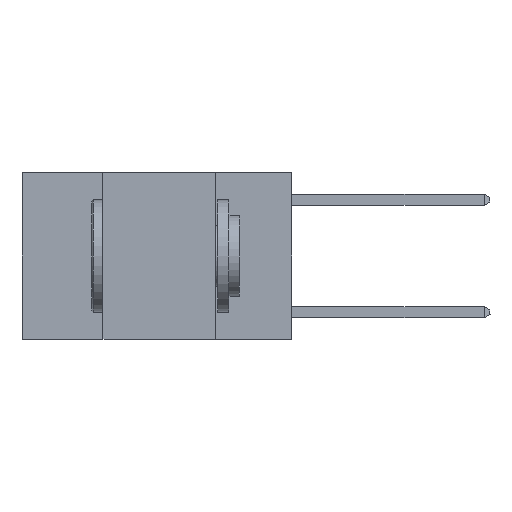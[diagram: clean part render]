
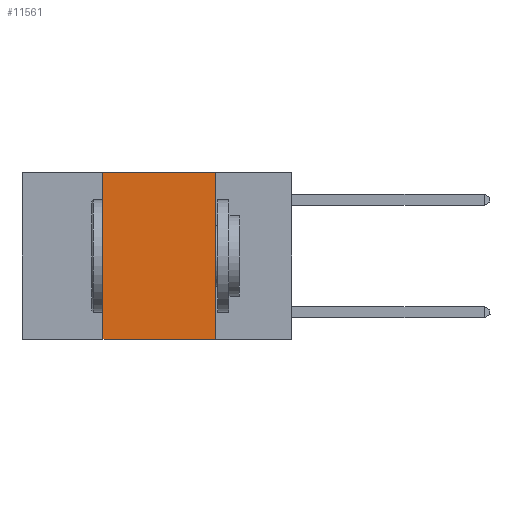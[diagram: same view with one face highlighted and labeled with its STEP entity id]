
A CAD part, left-side view. The second image highlights one B-rep face of the part: STEP entity #11561.
In plain terms, the highlighted planar face has unit normal (-1, 0, 0).
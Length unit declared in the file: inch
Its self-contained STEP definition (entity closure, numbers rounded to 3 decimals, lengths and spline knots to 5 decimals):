
#420 = CARTESIAN_POINT ( 'NONE',  ( 0., 0.17, 0. ) ) ;
#459 = VECTOR ( 'NONE', #11832, 39.37008 ) ;
#2336 = VERTEX_POINT ( 'NONE', #12070 ) ;
#3732 = EDGE_CURVE ( 'NONE', #14164, #17976, #16813, .T. ) ;
#5002 = AXIS2_PLACEMENT_3D ( 'NONE', #11891, #9206, #7597 ) ;
#5497 = CARTESIAN_POINT ( 'NONE',  ( 0., 0.42, 0. ) ) ;
#5906 = VECTOR ( 'NONE', #8807, 39.37008 ) ;
#6145 = PLANE ( 'NONE',  #5002 ) ;
#7201 = CARTESIAN_POINT ( 'NONE',  ( 0., 0.6, 0. ) ) ;
#7386 = DIRECTION ( 'NONE',  ( 0., -1., 0. ) ) ;
#7597 = DIRECTION ( 'NONE',  ( 0., 0., -1. ) ) ;
#7913 = VECTOR ( 'NONE', #7386, 39.37008 ) ;
#8432 = EDGE_CURVE ( 'NONE', #14164, #11278, #11641, .T. ) ;
#8807 = DIRECTION ( 'NONE',  ( 0., 0., -1. ) ) ;
#9206 = DIRECTION ( 'NONE',  ( 1., 0., 0. ) ) ;
#9426 = CARTESIAN_POINT ( 'NONE',  ( 0., 0.17, -0.37 ) ) ;
#9596 = CARTESIAN_POINT ( 'NONE',  ( 0., 0.42, 0. ) ) ;
#10205 = ORIENTED_EDGE ( 'NONE', *, *, #8432, .T. ) ;
#10263 = LINE ( 'NONE', #7201, #7913 ) ;
#10743 = EDGE_CURVE ( 'NONE', #2336, #11278, #14515, .T. ) ;
#11278 = VERTEX_POINT ( 'NONE', #9426 ) ;
#11561 = ADVANCED_FACE ( 'NONE', ( #11802 ), #6145, .F. ) ;
#11641 = LINE ( 'NONE', #14571, #459 ) ;
#11802 = FACE_OUTER_BOUND ( 'NONE', #14171, .T. ) ;
#11832 = DIRECTION ( 'NONE',  ( 0., -1., 0. ) ) ;
#11891 = CARTESIAN_POINT ( 'NONE',  ( 0., 0.6, 0. ) ) ;
#12070 = CARTESIAN_POINT ( 'NONE',  ( 0., 0.17, 0. ) ) ;
#13756 = CARTESIAN_POINT ( 'NONE',  ( 0., 0.42, -0.37 ) ) ;
#14053 = EDGE_CURVE ( 'NONE', #17976, #2336, #10263, .T. ) ;
#14164 = VERTEX_POINT ( 'NONE', #13756 ) ;
#14171 = EDGE_LOOP ( 'NONE', ( #18699, #14639, #18086, #10205 ) ) ;
#14515 = LINE ( 'NONE', #420, #5906 ) ;
#14571 = CARTESIAN_POINT ( 'NONE',  ( 0., 0.6, -0.37 ) ) ;
#14639 = ORIENTED_EDGE ( 'NONE', *, *, #14053, .F. ) ;
#16813 = LINE ( 'NONE', #9596, #18099 ) ;
#17976 = VERTEX_POINT ( 'NONE', #5497 ) ;
#18086 = ORIENTED_EDGE ( 'NONE', *, *, #3732, .F. ) ;
#18099 = VECTOR ( 'NONE', #18449, 39.37008 ) ;
#18449 = DIRECTION ( 'NONE',  ( 0., 0., 1. ) ) ;
#18699 = ORIENTED_EDGE ( 'NONE', *, *, #10743, .F. ) ;
